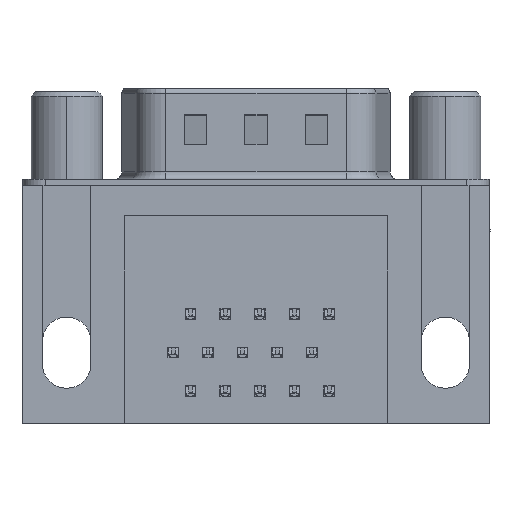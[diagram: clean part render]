
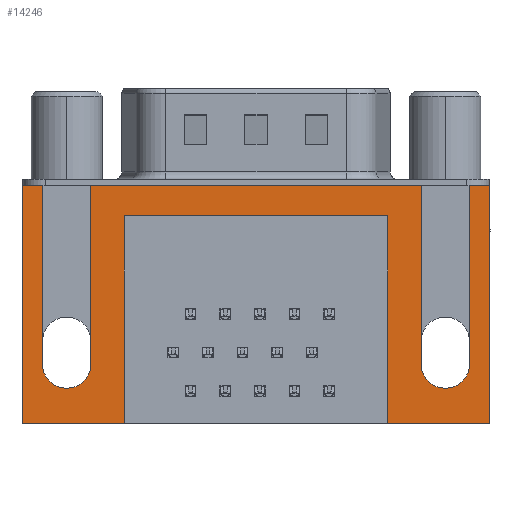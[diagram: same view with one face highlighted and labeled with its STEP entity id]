
A CAD part, front view. The second image highlights one B-rep face of the part: STEP entity #14246.
In plain terms, the highlighted planar face has unit normal (0, -1, 0).
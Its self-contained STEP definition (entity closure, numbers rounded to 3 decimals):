
#107 = VERTEX_POINT ( 'NONE', #20798 ) ;
#114 = VECTOR ( 'NONE', #18319, 1000. ) ;
#144 = ORIENTED_EDGE ( 'NONE', *, *, #6523, .F. ) ;
#151 = CARTESIAN_POINT ( 'NONE',  ( 23.39, -6.275, -11.78 ) ) ;
#186 = CARTESIAN_POINT ( 'NONE',  ( -2.91, -6.275, 0. ) ) ;
#387 = VECTOR ( 'NONE', #4334, 1000. ) ;
#400 = VERTEX_POINT ( 'NONE', #2017 ) ;
#409 = LINE ( 'NONE', #3061, #5151 ) ;
#433 = ORIENTED_EDGE ( 'NONE', *, *, #6126, .T. ) ;
#671 = DIRECTION ( 'NONE',  ( 0., -1., 0. ) ) ;
#896 = VECTOR ( 'NONE', #9152, 1000. ) ;
#1237 = VERTEX_POINT ( 'NONE', #14765 ) ;
#1278 = DIRECTION ( 'NONE',  ( 0., 0., 1. ) ) ;
#1581 = DIRECTION ( 'NONE',  ( 0., -1., 0. ) ) ;
#1917 = ORIENTED_EDGE ( 'NONE', *, *, #6496, .F. ) ;
#1938 = AXIS2_PLACEMENT_3D ( 'NONE', #2234, #9763, #16592 ) ;
#2017 = CARTESIAN_POINT ( 'NONE',  ( 3.79, -6.275, -2. ) ) ;
#2234 = CARTESIAN_POINT ( 'NONE',  ( 24.99, -6.275, -11.78 ) ) ;
#2265 = DIRECTION ( 'NONE',  ( 0., 0., -1. ) ) ;
#2278 = ORIENTED_EDGE ( 'NONE', *, *, #19027, .F. ) ;
#2323 = ORIENTED_EDGE ( 'NONE', *, *, #18974, .F. ) ;
#2523 = VERTEX_POINT ( 'NONE', #21963 ) ;
#2637 = CARTESIAN_POINT ( 'NONE',  ( 27.9, -6.275, -15.7 ) ) ;
#2752 = ORIENTED_EDGE ( 'NONE', *, *, #6468, .F. ) ;
#2978 = FACE_OUTER_BOUND ( 'NONE', #4260, .T. ) ;
#3061 = CARTESIAN_POINT ( 'NONE',  ( -2.91, -6.275, -2.5 ) ) ;
#3294 = VERTEX_POINT ( 'NONE', #17363 ) ;
#3429 = CIRCLE ( 'NONE', #11508, 1.6 ) ;
#3523 = VERTEX_POINT ( 'NONE', #18086 ) ;
#3661 = LINE ( 'NONE', #8427, #11805 ) ;
#4004 = DIRECTION ( 'NONE',  ( 0., 0., -1. ) ) ;
#4118 = CARTESIAN_POINT ( 'NONE',  ( 0., -6.275, -11.78 ) ) ;
#4163 = CIRCLE ( 'NONE', #11227, 1.6 ) ;
#4260 = EDGE_LOOP ( 'NONE', ( #13313, #2323, #11681, #20400, #19734, #5408, #2278, #9290, #6605, #2752, #4936, #1917, #6535, #22001, #16577, #144, #433, #16846 ) ) ;
#4334 = DIRECTION ( 'NONE',  ( 1., 0., 0. ) ) ;
#4618 = LINE ( 'NONE', #12489, #21265 ) ;
#4936 = ORIENTED_EDGE ( 'NONE', *, *, #5631, .F. ) ;
#5018 = CARTESIAN_POINT ( 'NONE',  ( 23.39, -6.275, 0. ) ) ;
#5133 = VECTOR ( 'NONE', #19975, 1000. ) ;
#5151 = VECTOR ( 'NONE', #18196, 1000. ) ;
#5408 = ORIENTED_EDGE ( 'NONE', *, *, #6415, .F. ) ;
#5631 = EDGE_CURVE ( 'NONE', #5885, #1237, #409, .T. ) ;
#5668 = DIRECTION ( 'NONE',  ( 0., 0., -1. ) ) ;
#5885 = VERTEX_POINT ( 'NONE', #13194 ) ;
#6126 = EDGE_CURVE ( 'NONE', #14652, #15208, #8624, .T. ) ;
#6266 = EDGE_CURVE ( 'NONE', #14328, #20055, #7587, .T. ) ;
#6290 = EDGE_CURVE ( 'NONE', #20714, #15895, #11019, .T. ) ;
#6342 = EDGE_CURVE ( 'NONE', #15022, #20714, #16019, .T. ) ;
#6379 = EDGE_CURVE ( 'NONE', #3294, #15022, #14383, .T. ) ;
#6394 = VERTEX_POINT ( 'NONE', #10447 ) ;
#6415 = EDGE_CURVE ( 'NONE', #19329, #3294, #9422, .T. ) ;
#6419 = VERTEX_POINT ( 'NONE', #16606 ) ;
#6442 = EDGE_CURVE ( 'NONE', #107, #6419, #17995, .T. ) ;
#6468 = EDGE_CURVE ( 'NONE', #1237, #107, #13346, .T. ) ;
#6496 = EDGE_CURVE ( 'NONE', #15228, #5885, #21875, .T. ) ;
#6500 = EDGE_CURVE ( 'NONE', #400, #15228, #7816, .T. ) ;
#6518 = EDGE_CURVE ( 'NONE', #3523, #400, #4618, .T. ) ;
#6523 = EDGE_CURVE ( 'NONE', #14652, #2523, #3661, .T. ) ;
#6535 = ORIENTED_EDGE ( 'NONE', *, *, #6500, .F. ) ;
#6554 = EDGE_CURVE ( 'NONE', #2523, #3523, #16305, .T. ) ;
#6605 = ORIENTED_EDGE ( 'NONE', *, *, #6442, .F. ) ;
#7587 = LINE ( 'NONE', #15061, #20350 ) ;
#7816 = LINE ( 'NONE', #18749, #16867 ) ;
#8306 = CARTESIAN_POINT ( 'NONE',  ( 1.6, -6.275, -11.78 ) ) ;
#8427 = CARTESIAN_POINT ( 'NONE',  ( 27.9, -6.275, -15.7 ) ) ;
#8624 = LINE ( 'NONE', #18337, #114 ) ;
#8866 = VECTOR ( 'NONE', #4004, 1000. ) ;
#9152 = DIRECTION ( 'NONE',  ( 0., 0., 1. ) ) ;
#9290 = ORIENTED_EDGE ( 'NONE', *, *, #18872, .F. ) ;
#9305 = CARTESIAN_POINT ( 'NONE',  ( -1.6, -6.275, 0. ) ) ;
#9358 = EDGE_CURVE ( 'NONE', #20055, #15208, #19908, .T. ) ;
#9420 = CARTESIAN_POINT ( 'NONE',  ( 24.99, -6.275, -11.78 ) ) ;
#9422 = LINE ( 'NONE', #10265, #896 ) ;
#9533 = CARTESIAN_POINT ( 'NONE',  ( 27.9, -6.275, -15.7 ) ) ;
#9763 = DIRECTION ( 'NONE',  ( 0., -1., 0. ) ) ;
#9843 = DIRECTION ( 'NONE',  ( 1., 0., 0. ) ) ;
#9847 = DIRECTION ( 'NONE',  ( 1., 0., 0. ) ) ;
#10265 = CARTESIAN_POINT ( 'NONE',  ( 1.6, -6.275, 0. ) ) ;
#10316 = CARTESIAN_POINT ( 'NONE',  ( -2.91, -6.275, -2.5 ) ) ;
#10447 = CARTESIAN_POINT ( 'NONE',  ( 0., -6.275, -13.38 ) ) ;
#10530 = CARTESIAN_POINT ( 'NONE',  ( 21.2, -6.275, -2. ) ) ;
#11019 = CIRCLE ( 'NONE', #1938, 1.6 ) ;
#11122 = DIRECTION ( 'NONE',  ( 0., 0., 1. ) ) ;
#11191 = AXIS2_PLACEMENT_3D ( 'NONE', #11268, #1581, #12941 ) ;
#11227 = AXIS2_PLACEMENT_3D ( 'NONE', #9420, #21786, #11122 ) ;
#11268 = CARTESIAN_POINT ( 'NONE',  ( 0., -6.275, -11.78 ) ) ;
#11508 = AXIS2_PLACEMENT_3D ( 'NONE', #4118, #15595, #5668 ) ;
#11681 = ORIENTED_EDGE ( 'NONE', *, *, #6290, .F. ) ;
#11703 = DIRECTION ( 'NONE',  ( -1., 0., 0. ) ) ;
#11805 = VECTOR ( 'NONE', #11703, 1000. ) ;
#11925 = CARTESIAN_POINT ( 'NONE',  ( -2.91, -6.275, 0. ) ) ;
#12035 = DIRECTION ( 'NONE',  ( 0., 0., -1. ) ) ;
#12419 = CARTESIAN_POINT ( 'NONE',  ( 26.59, -6.275, 0. ) ) ;
#12489 = CARTESIAN_POINT ( 'NONE',  ( 3.79, -6.275, -2. ) ) ;
#12941 = DIRECTION ( 'NONE',  ( 0., 0., -1. ) ) ;
#13194 = CARTESIAN_POINT ( 'NONE',  ( -2.91, -6.275, -15.7 ) ) ;
#13313 = ORIENTED_EDGE ( 'NONE', *, *, #6266, .F. ) ;
#13346 = LINE ( 'NONE', #11925, #387 ) ;
#13598 = PLANE ( 'NONE',  #19095 ) ;
#13660 = CARTESIAN_POINT ( 'NONE',  ( 26.59, -6.275, -11.78 ) ) ;
#14246 = ADVANCED_FACE ( 'NONE', ( #2978 ), #13598, .T. ) ;
#14328 = VERTEX_POINT ( 'NONE', #13660 ) ;
#14383 = LINE ( 'NONE', #21506, #18584 ) ;
#14425 = DIRECTION ( 'NONE',  ( 0., 0., -1. ) ) ;
#14652 = VERTEX_POINT ( 'NONE', #2637 ) ;
#14765 = CARTESIAN_POINT ( 'NONE',  ( -2.91, -6.275, 0. ) ) ;
#15022 = VERTEX_POINT ( 'NONE', #5018 ) ;
#15040 = VECTOR ( 'NONE', #9843, 1000. ) ;
#15061 = CARTESIAN_POINT ( 'NONE',  ( 26.59, -6.275, 0. ) ) ;
#15172 = DIRECTION ( 'NONE',  ( -1., 0., 0. ) ) ;
#15208 = VERTEX_POINT ( 'NONE', #20908 ) ;
#15228 = VERTEX_POINT ( 'NONE', #15411 ) ;
#15411 = CARTESIAN_POINT ( 'NONE',  ( 3.79, -6.275, -15.7 ) ) ;
#15595 = DIRECTION ( 'NONE',  ( 0., -1., 0. ) ) ;
#15735 = CIRCLE ( 'NONE', #11191, 1.6 ) ;
#15895 = VERTEX_POINT ( 'NONE', #18296 ) ;
#16019 = LINE ( 'NONE', #16664, #19179 ) ;
#16150 = DIRECTION ( 'NONE',  ( 0., 0., 1. ) ) ;
#16305 = LINE ( 'NONE', #10530, #20636 ) ;
#16577 = ORIENTED_EDGE ( 'NONE', *, *, #6554, .F. ) ;
#16592 = DIRECTION ( 'NONE',  ( 0., 0., 1. ) ) ;
#16606 = CARTESIAN_POINT ( 'NONE',  ( -1.6, -6.275, -11.78 ) ) ;
#16664 = CARTESIAN_POINT ( 'NONE',  ( 23.39, -6.275, 0. ) ) ;
#16846 = ORIENTED_EDGE ( 'NONE', *, *, #9358, .F. ) ;
#16867 = VECTOR ( 'NONE', #2265, 1000. ) ;
#17363 = CARTESIAN_POINT ( 'NONE',  ( 1.6, -6.275, 0. ) ) ;
#17995 = LINE ( 'NONE', #9305, #8866 ) ;
#18086 = CARTESIAN_POINT ( 'NONE',  ( 21.2, -6.275, -2. ) ) ;
#18196 = DIRECTION ( 'NONE',  ( 0., 0., 1. ) ) ;
#18296 = CARTESIAN_POINT ( 'NONE',  ( 24.99, -6.275, -13.38 ) ) ;
#18319 = DIRECTION ( 'NONE',  ( 0., 0., 1. ) ) ;
#18337 = CARTESIAN_POINT ( 'NONE',  ( 27.9, -6.275, -2.5 ) ) ;
#18584 = VECTOR ( 'NONE', #9847, 1000. ) ;
#18749 = CARTESIAN_POINT ( 'NONE',  ( 3.79, -6.275, -2. ) ) ;
#18872 = EDGE_CURVE ( 'NONE', #6419, #6394, #3429, .T. ) ;
#18974 = EDGE_CURVE ( 'NONE', #15895, #14328, #4163, .T. ) ;
#19027 = EDGE_CURVE ( 'NONE', #6394, #19329, #15735, .T. ) ;
#19095 = AXIS2_PLACEMENT_3D ( 'NONE', #10316, #671, #12035 ) ;
#19179 = VECTOR ( 'NONE', #14425, 1000. ) ;
#19329 = VERTEX_POINT ( 'NONE', #8306 ) ;
#19734 = ORIENTED_EDGE ( 'NONE', *, *, #6379, .F. ) ;
#19908 = LINE ( 'NONE', #186, #15040 ) ;
#19975 = DIRECTION ( 'NONE',  ( -1., 0., 0. ) ) ;
#20055 = VERTEX_POINT ( 'NONE', #12419 ) ;
#20350 = VECTOR ( 'NONE', #16150, 1000. ) ;
#20400 = ORIENTED_EDGE ( 'NONE', *, *, #6342, .F. ) ;
#20636 = VECTOR ( 'NONE', #1278, 1000. ) ;
#20714 = VERTEX_POINT ( 'NONE', #151 ) ;
#20798 = CARTESIAN_POINT ( 'NONE',  ( -1.6, -6.275, 0. ) ) ;
#20908 = CARTESIAN_POINT ( 'NONE',  ( 27.9, -6.275, 0. ) ) ;
#21265 = VECTOR ( 'NONE', #15172, 1000. ) ;
#21506 = CARTESIAN_POINT ( 'NONE',  ( -2.91, -6.275, 0. ) ) ;
#21786 = DIRECTION ( 'NONE',  ( 0., -1., 0. ) ) ;
#21875 = LINE ( 'NONE', #9533, #5133 ) ;
#21963 = CARTESIAN_POINT ( 'NONE',  ( 21.2, -6.275, -15.7 ) ) ;
#22001 = ORIENTED_EDGE ( 'NONE', *, *, #6518, .F. ) ;
